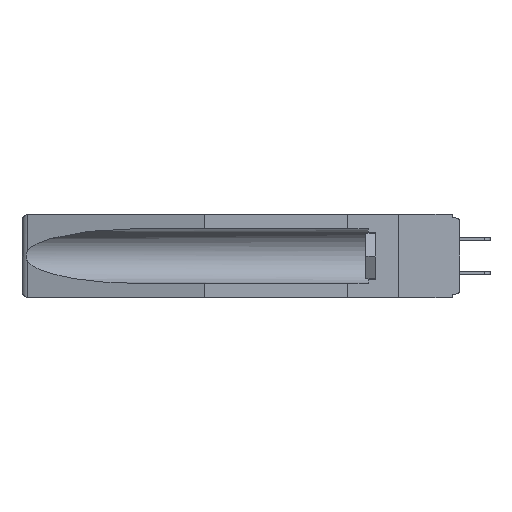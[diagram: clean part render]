
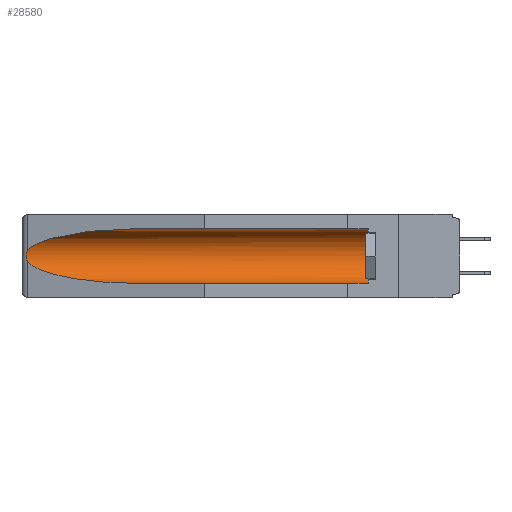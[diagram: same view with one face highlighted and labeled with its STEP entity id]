
A CAD part, left-side view. The second image highlights one B-rep face of the part: STEP entity #28580.
In plain terms, the highlighted cylindrical face has radius 2.857 mm (diameter 5.715 mm), a partial arc.
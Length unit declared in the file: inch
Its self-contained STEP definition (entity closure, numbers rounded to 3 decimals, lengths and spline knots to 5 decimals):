
#349 = CARTESIAN_POINT ( 'NONE',  ( 0.155, 0.126, -0.284 ) ) ;
#383 = VECTOR ( 'NONE', #15638, 39.37008 ) ;
#431 = VERTEX_POINT ( 'NONE', #13906 ) ;
#689 = CARTESIAN_POINT ( 'NONE',  ( 0.25451, 1.48313, -0.24835 ) ) ;
#860 = EDGE_CURVE ( 'NONE', #3011, #23188, #11389, .T. ) ;
#1170 = EDGE_LOOP ( 'NONE', ( #18288, #20247, #22756, #13497, #19216, #23618 ) ) ;
#1327 = CARTESIAN_POINT ( 'NONE',  ( 0.155, 1.07973, -0.284 ) ) ;
#1681 = CARTESIAN_POINT ( 'NONE',  ( 0.2675, 1.53308, -0.17534 ) ) ;
#1882 = CARTESIAN_POINT ( 'NONE',  ( 0.26537, 1.52718, -0.19328 ) ) ;
#2328 = CARTESIAN_POINT ( 'NONE',  ( 0.26537, 1.52718, -0.14972 ) ) ;
#2781 = CARTESIAN_POINT ( 'NONE',  ( 0.26537, 1.52718, -0.19328 ) ) ;
#3011 = VERTEX_POINT ( 'NONE', #349 ) ;
#3761 = CARTESIAN_POINT ( 'NONE',  ( 0.2673, 1.53269, -0.17917 ) ) ;
#3823 =( BOUNDED_CURVE ( )  B_SPLINE_CURVE ( 3, ( #2781, #689, #23593, #4960 ),
 .UNSPECIFIED., .F., .F. ) 
 B_SPLINE_CURVE_WITH_KNOTS ( ( 4, 4 ),
 ( 0.1948, 1.5708 ),
 .UNSPECIFIED. ) 
 CURVE ( )  GEOMETRIC_REPRESENTATION_ITEM ( )  RATIONAL_B_SPLINE_CURVE ( ( 1., 0.848, 0.848, 1. ) ) 
 REPRESENTATION_ITEM ( '' )  );
#4159 = CARTESIAN_POINT ( 'NONE',  ( 0.26654, 1.53092, -0.15636 ) ) ;
#4939 = DIRECTION ( 'NONE',  ( 0., 0., 1. ) ) ;
#4960 = CARTESIAN_POINT ( 'NONE',  ( 0.155, 1.07973, -0.284 ) ) ;
#6509 = CARTESIAN_POINT ( 'NONE',  ( 0.155, 1.07973, -0.059 ) ) ;
#6643 = EDGE_CURVE ( 'NONE', #12989, #431, #17146, .T. ) ;
#7036 = LINE ( 'NONE', #7128, #23091 ) ;
#7128 = CARTESIAN_POINT ( 'NONE',  ( 0.155, -0.30754, -0.059 ) ) ;
#7424 = CARTESIAN_POINT ( 'NONE',  ( 0.155, 0.126, -0.1715 ) ) ;
#7939 = DIRECTION ( 'NONE',  ( 0., 0., 1. ) ) ;
#8730 = CARTESIAN_POINT ( 'NONE',  ( 0.155, -0.30754, -0.284 ) ) ;
#9948 = CARTESIAN_POINT ( 'NONE',  ( 0.21114, 1.30732, -0.059 ) ) ;
#10248 = CARTESIAN_POINT ( 'NONE',  ( 0.25451, 1.48313, -0.09465 ) ) ;
#10633 = CARTESIAN_POINT ( 'NONE',  ( 0.26537, 1.52718, -0.14972 ) ) ;
#11389 = LINE ( 'NONE', #8730, #383 ) ;
#11392 = VERTEX_POINT ( 'NONE', #26426 ) ;
#12989 = VERTEX_POINT ( 'NONE', #2328 ) ;
#13230 = CARTESIAN_POINT ( 'NONE',  ( 0.2675, 1.53308, -0.16763 ) ) ;
#13497 = ORIENTED_EDGE ( 'NONE', *, *, #860, .F. ) ;
#13906 = CARTESIAN_POINT ( 'NONE',  ( 0.26537, 1.52718, -0.19328 ) ) ;
#14543 = CARTESIAN_POINT ( 'NONE',  ( 0.26537, 1.52718, -0.14972 ) ) ;
#15346 =( BOUNDED_CURVE ( )  B_SPLINE_CURVE ( 3, ( #24003, #9948, #10248, #14543 ),
 .UNSPECIFIED., .F., .F. ) 
 B_SPLINE_CURVE_WITH_KNOTS ( ( 4, 4 ),
 ( 4.71239, 6.08839 ),
 .UNSPECIFIED. ) 
 CURVE ( )  GEOMETRIC_REPRESENTATION_ITEM ( )  RATIONAL_B_SPLINE_CURVE ( ( 1., 0.848, 0.848, 1. ) ) 
 REPRESENTATION_ITEM ( '' )  );
#15522 = CARTESIAN_POINT ( 'NONE',  ( 0.26597, 1.5296, -0.19026 ) ) ;
#15600 = CIRCLE ( 'NONE', #22171, 0.1125 ) ;
#15638 = DIRECTION ( 'NONE',  ( 0., 1., 0. ) ) ;
#16300 = DIRECTION ( 'NONE',  ( 0., 1., 0. ) ) ;
#16313 = VERTEX_POINT ( 'NONE', #6509 ) ;
#16755 = CYLINDRICAL_SURFACE ( 'NONE', #20104, 0.1125 ) ;
#16851 = EDGE_CURVE ( 'NONE', #16313, #12989, #15346, .T. ) ;
#17016 = CARTESIAN_POINT ( 'NONE',  ( 0.155, -0.30754, -0.1715 ) ) ;
#17146 = B_SPLINE_CURVE_WITH_KNOTS ( 'NONE', 3,
 ( #10633, #20014, #4159, #22297, #13230, #1681, #3761, #29198, #15522, #1882 ),
 .UNSPECIFIED., .F., .F.,
 ( 4, 2, 2, 2, 4 ),
 ( 0., 0.00029, 0.00058, 0.00087, 0.00117 ),
 .UNSPECIFIED. ) ;
#17779 = EDGE_CURVE ( 'NONE', #431, #23188, #3823, .T. ) ;
#18288 = ORIENTED_EDGE ( 'NONE', *, *, #16851, .T. ) ;
#18480 = DIRECTION ( 'NONE',  ( 0., -1., 0. ) ) ;
#19216 = ORIENTED_EDGE ( 'NONE', *, *, #23411, .T. ) ;
#20014 = CARTESIAN_POINT ( 'NONE',  ( 0.26597, 1.52961, -0.15275 ) ) ;
#20104 = AXIS2_PLACEMENT_3D ( 'NONE', #17016, #21615, #7939 ) ;
#20247 = ORIENTED_EDGE ( 'NONE', *, *, #6643, .T. ) ;
#21615 = DIRECTION ( 'NONE',  ( 0., 1., 0. ) ) ;
#22171 = AXIS2_PLACEMENT_3D ( 'NONE', #7424, #18480, #4939 ) ;
#22297 = CARTESIAN_POINT ( 'NONE',  ( 0.2673, 1.5327, -0.16383 ) ) ;
#22756 = ORIENTED_EDGE ( 'NONE', *, *, #17779, .T. ) ;
#23091 = VECTOR ( 'NONE', #16300, 39.37008 ) ;
#23188 = VERTEX_POINT ( 'NONE', #1327 ) ;
#23411 = EDGE_CURVE ( 'NONE', #3011, #11392, #15600, .T. ) ;
#23454 = EDGE_CURVE ( 'NONE', #11392, #16313, #7036, .T. ) ;
#23593 = CARTESIAN_POINT ( 'NONE',  ( 0.21114, 1.30732, -0.284 ) ) ;
#23618 = ORIENTED_EDGE ( 'NONE', *, *, #23454, .T. ) ;
#24003 = CARTESIAN_POINT ( 'NONE',  ( 0.155, 1.07973, -0.059 ) ) ;
#26062 = FACE_OUTER_BOUND ( 'NONE', #1170, .T. ) ;
#26426 = CARTESIAN_POINT ( 'NONE',  ( 0.155, 0.126, -0.059 ) ) ;
#28580 = ADVANCED_FACE ( 'NONE', ( #26062 ), #16755, .F. ) ;
#29198 = CARTESIAN_POINT ( 'NONE',  ( 0.26655, 1.53094, -0.18657 ) ) ;
